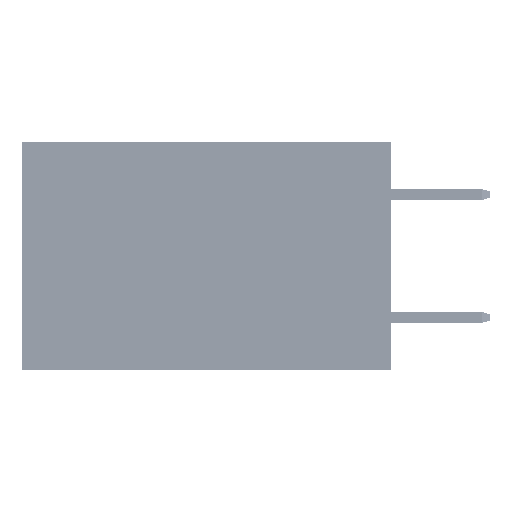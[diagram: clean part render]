
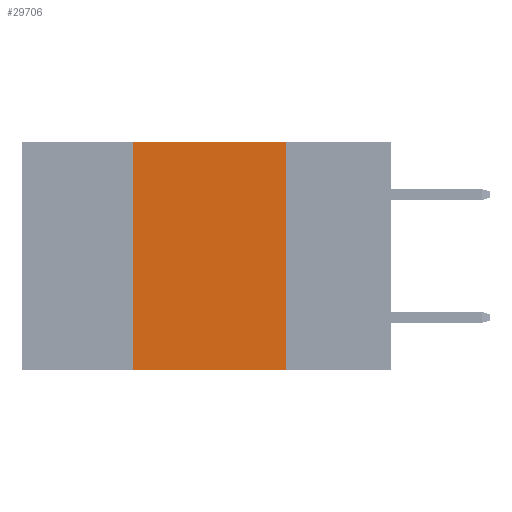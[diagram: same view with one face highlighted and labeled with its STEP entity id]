
A CAD part, left-side view. The second image highlights one B-rep face of the part: STEP entity #29706.
In plain terms, the highlighted planar face has unit normal (-1, 0, 0).
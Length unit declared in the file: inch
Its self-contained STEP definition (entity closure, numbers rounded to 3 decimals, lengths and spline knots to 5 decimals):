
#3383 = LINE ( 'NONE', #40899, #28692 ) ;
#5409 = VERTEX_POINT ( 'NONE', #35834 ) ;
#5422 = CARTESIAN_POINT ( 'NONE',  ( 0., 0.42, -0.37 ) ) ;
#7883 = DIRECTION ( 'NONE',  ( 0., 0., -1. ) ) ;
#8901 = LINE ( 'NONE', #27772, #19475 ) ;
#9206 = CARTESIAN_POINT ( 'NONE',  ( 0., 0.17, -0.37 ) ) ;
#9567 = DIRECTION ( 'NONE',  ( 1., 0., 0. ) ) ;
#10890 = DIRECTION ( 'NONE',  ( 0., 0., 1. ) ) ;
#13209 = PLANE ( 'NONE',  #33905 ) ;
#17294 = CARTESIAN_POINT ( 'NONE',  ( 0., 0.6, 0. ) ) ;
#19475 = VECTOR ( 'NONE', #43123, 39.37008 ) ;
#21112 = DIRECTION ( 'NONE',  ( 0., 0., -1. ) ) ;
#21986 = FACE_OUTER_BOUND ( 'NONE', #37283, .T. ) ;
#22145 = VERTEX_POINT ( 'NONE', #9206 ) ;
#24985 = CARTESIAN_POINT ( 'NONE',  ( 0., 0.42, 0. ) ) ;
#25230 = VECTOR ( 'NONE', #10890, 39.37008 ) ;
#26984 = VERTEX_POINT ( 'NONE', #24985 ) ;
#27424 = ORIENTED_EDGE ( 'NONE', *, *, #36594, .F. ) ;
#27772 = CARTESIAN_POINT ( 'NONE',  ( 0., 0.6, 0. ) ) ;
#28692 = VECTOR ( 'NONE', #48476, 39.37008 ) ;
#29357 = LINE ( 'NONE', #30314, #25230 ) ;
#29706 = ADVANCED_FACE ( 'NONE', ( #21986 ), #13209, .F. ) ;
#30064 = LINE ( 'NONE', #37546, #34180 ) ;
#30188 = ORIENTED_EDGE ( 'NONE', *, *, #48515, .T. ) ;
#30314 = CARTESIAN_POINT ( 'NONE',  ( 0., 0.42, 0. ) ) ;
#33120 = EDGE_CURVE ( 'NONE', #33444, #26984, #29357, .T. ) ;
#33444 = VERTEX_POINT ( 'NONE', #5422 ) ;
#33905 = AXIS2_PLACEMENT_3D ( 'NONE', #17294, #9567, #21112 ) ;
#34180 = VECTOR ( 'NONE', #7883, 39.37008 ) ;
#35834 = CARTESIAN_POINT ( 'NONE',  ( 0., 0.17, 0. ) ) ;
#36594 = EDGE_CURVE ( 'NONE', #26984, #5409, #8901, .T. ) ;
#36896 = EDGE_CURVE ( 'NONE', #5409, #22145, #30064, .T. ) ;
#37283 = EDGE_LOOP ( 'NONE', ( #41119, #27424, #43934, #30188 ) ) ;
#37546 = CARTESIAN_POINT ( 'NONE',  ( 0., 0.17, 0. ) ) ;
#40899 = CARTESIAN_POINT ( 'NONE',  ( 0., 0.6, -0.37 ) ) ;
#41119 = ORIENTED_EDGE ( 'NONE', *, *, #36896, .F. ) ;
#43123 = DIRECTION ( 'NONE',  ( 0., -1., 0. ) ) ;
#43934 = ORIENTED_EDGE ( 'NONE', *, *, #33120, .F. ) ;
#48476 = DIRECTION ( 'NONE',  ( 0., -1., 0. ) ) ;
#48515 = EDGE_CURVE ( 'NONE', #33444, #22145, #3383, .T. ) ;
